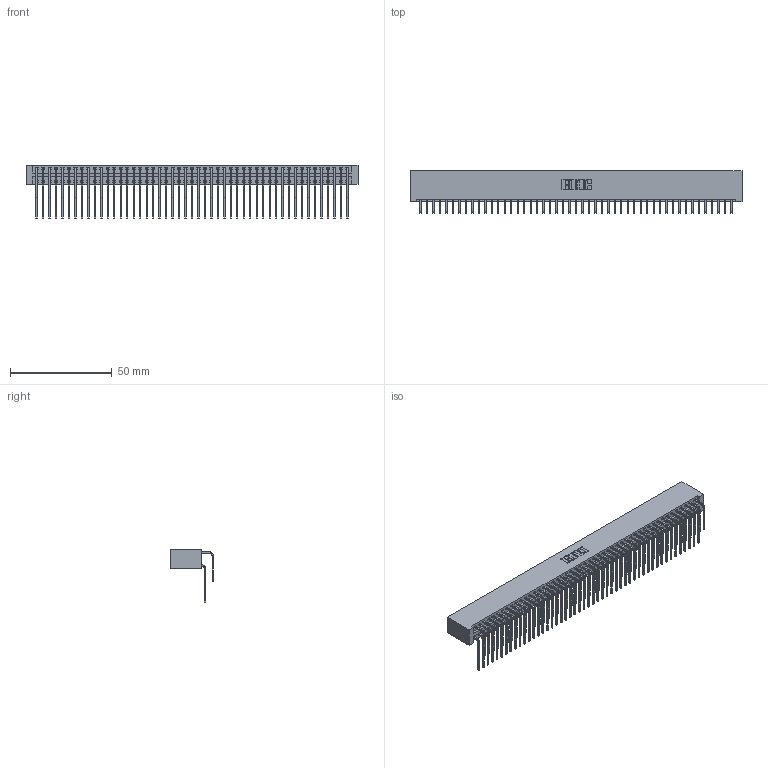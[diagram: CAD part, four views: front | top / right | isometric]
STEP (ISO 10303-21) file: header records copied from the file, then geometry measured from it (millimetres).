
FILE_DESCRIPTION (( 'STEP AP203' ), '1' );
FILE_NAME ('396-098-559-201.STEP', '2018-09-14T05:58:36', ( '' ), ( '' ), 'SwSTEP 2.0', 'SolidWorks 2016', '' );
FILE_SCHEMA (( 'CONFIG_CONTROL_DESIGN' ));
Length unit declared in the file: inch
Products named in the file (4): 346 Part_No Mounting Lugs; 345-292-001_558 559 Tail - 1; 345-292-001_559 Tail - 2; 396-098-559-201
Assembly tree (99 placements, depth 2):
  396-098-559-201
    346 Part_No Mounting Lugs
    345-292-001_558 559 Tail - 1  x49
    345-292-001_559 Tail - 2  x49
Bounding box: 162.81 x 20.89 x 26.16 mm (x, y, z)
Volume: 17069.4 mm3; surface area: 26448.3 mm2
Topology: 99 solids, 99 shells, 5406 faces, 16083 edges, 10590 vertices
Faces by surface type: plane 3698, cylinder 1708
Entity records: 32543 total; most frequent: CARTESIAN_POINT 5403, ORIENTED_EDGE 5286, DIRECTION 4779, EDGE_CURVE 2643, LINE 2283, VECTOR 2283, VERTEX_POINT 1758, AXIS2_PLACEMENT_3D 1248
